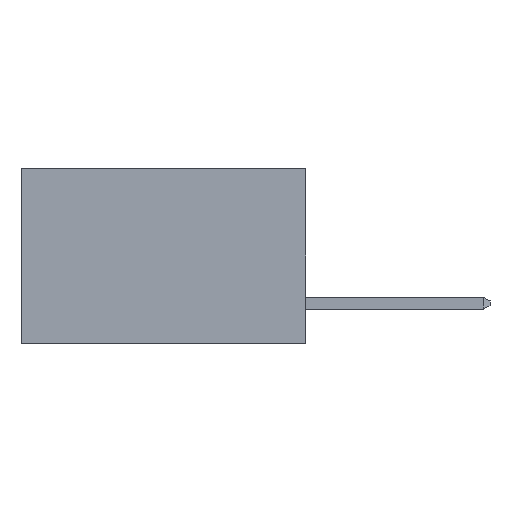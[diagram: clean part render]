
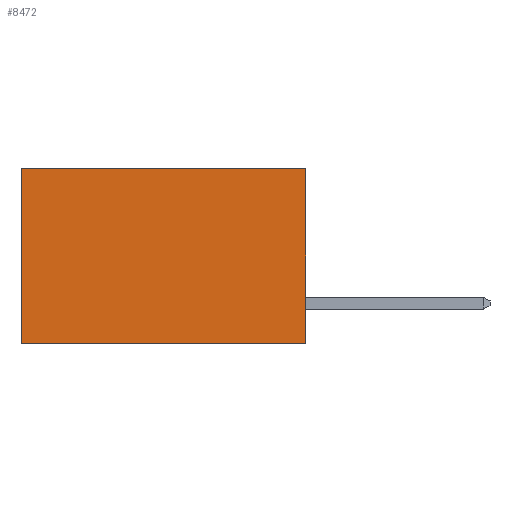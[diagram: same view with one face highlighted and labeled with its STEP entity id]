
A CAD part, left-side view. The second image highlights one B-rep face of the part: STEP entity #8472.
In plain terms, the highlighted planar face has unit normal (-1, 0, 0).
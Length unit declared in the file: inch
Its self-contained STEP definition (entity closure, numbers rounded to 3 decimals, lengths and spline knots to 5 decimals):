
#29 = VECTOR ( 'NONE', #10535, 39.37008 ) ;
#210 = EDGE_CURVE ( 'NONE', #417, #1902, #5871, .T. ) ;
#417 = VERTEX_POINT ( 'NONE', #6715 ) ;
#1058 = LINE ( 'NONE', #11595, #8932 ) ;
#1074 = AXIS2_PLACEMENT_3D ( 'NONE', #1414, #2476, #9562 ) ;
#1170 = CARTESIAN_POINT ( 'NONE',  ( 0.298, 0., -0.37 ) ) ;
#1291 = CARTESIAN_POINT ( 'NONE',  ( 0.298, 0., 0. ) ) ;
#1414 = CARTESIAN_POINT ( 'NONE',  ( 0.298, 0., 0. ) ) ;
#1454 = VERTEX_POINT ( 'NONE', #12417 ) ;
#1902 = VERTEX_POINT ( 'NONE', #9931 ) ;
#2476 = DIRECTION ( 'NONE',  ( 1., 0., 0. ) ) ;
#2505 = DIRECTION ( 'NONE',  ( 0., 0., -1. ) ) ;
#2590 = DIRECTION ( 'NONE',  ( 0., 1., 0. ) ) ;
#3985 = VECTOR ( 'NONE', #2505, 39.37008 ) ;
#4339 = LINE ( 'NONE', #7692, #3985 ) ;
#5155 = ORIENTED_EDGE ( 'NONE', *, *, #210, .T. ) ;
#5667 = CARTESIAN_POINT ( 'NONE',  ( 0.298, 0.6, 0. ) ) ;
#5672 = FACE_OUTER_BOUND ( 'NONE', #9102, .T. ) ;
#5865 = VECTOR ( 'NONE', #11414, 39.37008 ) ;
#5871 = LINE ( 'NONE', #5667, #29 ) ;
#6715 = CARTESIAN_POINT ( 'NONE',  ( 0.298, 0.6, 0. ) ) ;
#7085 = VERTEX_POINT ( 'NONE', #1170 ) ;
#7664 = PLANE ( 'NONE',  #1074 ) ;
#7669 = EDGE_CURVE ( 'NONE', #1454, #417, #8407, .T. ) ;
#7692 = CARTESIAN_POINT ( 'NONE',  ( 0.298, 0., 0. ) ) ;
#8407 = LINE ( 'NONE', #1291, #5865 ) ;
#8472 = ADVANCED_FACE ( 'NONE', ( #5672 ), #7664, .F. ) ;
#8932 = VECTOR ( 'NONE', #2590, 39.37008 ) ;
#8997 = EDGE_CURVE ( 'NONE', #1454, #7085, #4339, .T. ) ;
#9102 = EDGE_LOOP ( 'NONE', ( #5155, #10922, #11851, #11255 ) ) ;
#9562 = DIRECTION ( 'NONE',  ( 0., 0., -1. ) ) ;
#9931 = CARTESIAN_POINT ( 'NONE',  ( 0.298, 0.6, -0.37 ) ) ;
#10535 = DIRECTION ( 'NONE',  ( 0., 0., -1. ) ) ;
#10922 = ORIENTED_EDGE ( 'NONE', *, *, #11197, .F. ) ;
#11197 = EDGE_CURVE ( 'NONE', #7085, #1902, #1058, .T. ) ;
#11255 = ORIENTED_EDGE ( 'NONE', *, *, #7669, .T. ) ;
#11414 = DIRECTION ( 'NONE',  ( 0., 1., 0. ) ) ;
#11595 = CARTESIAN_POINT ( 'NONE',  ( 0.298, 0., -0.37 ) ) ;
#11851 = ORIENTED_EDGE ( 'NONE', *, *, #8997, .F. ) ;
#12417 = CARTESIAN_POINT ( 'NONE',  ( 0.298, 0., 0. ) ) ;
